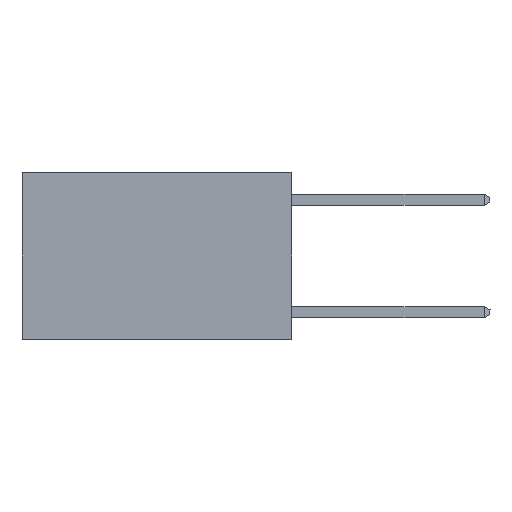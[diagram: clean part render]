
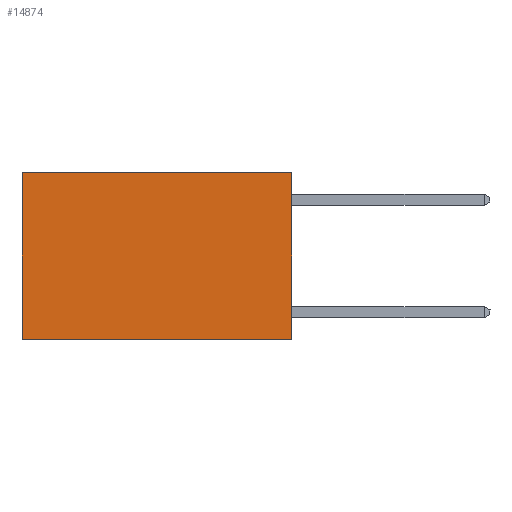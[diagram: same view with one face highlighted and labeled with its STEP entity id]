
A CAD part, left-side view. The second image highlights one B-rep face of the part: STEP entity #14874.
In plain terms, the highlighted planar face has unit normal (-1, 0, 0).
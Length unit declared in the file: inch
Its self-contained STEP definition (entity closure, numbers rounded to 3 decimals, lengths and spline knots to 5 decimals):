
#250 = CARTESIAN_POINT ( 'NONE',  ( 0.2625, 0., -0.37 ) ) ;
#368 = AXIS2_PLACEMENT_3D ( 'NONE', #15820, #8457, #18612 ) ;
#1188 = CARTESIAN_POINT ( 'NONE',  ( 0.2625, 0., 0. ) ) ;
#1323 = VERTEX_POINT ( 'NONE', #18005 ) ;
#1894 = VERTEX_POINT ( 'NONE', #3843 ) ;
#2519 = EDGE_CURVE ( 'NONE', #1323, #7548, #11680, .T. ) ;
#2812 = DIRECTION ( 'NONE',  ( 0., 0., -1. ) ) ;
#2916 = FACE_OUTER_BOUND ( 'NONE', #14482, .T. ) ;
#3797 = LINE ( 'NONE', #1188, #12005 ) ;
#3843 = CARTESIAN_POINT ( 'NONE',  ( 0.2625, 0.6, -0.37 ) ) ;
#4277 = VECTOR ( 'NONE', #8783, 39.37008 ) ;
#4704 = DIRECTION ( 'NONE',  ( 0., 1., 0. ) ) ;
#6889 = PLANE ( 'NONE',  #368 ) ;
#7424 = EDGE_CURVE ( 'NONE', #7548, #1894, #12476, .T. ) ;
#7445 = EDGE_CURVE ( 'NONE', #1323, #9102, #3797, .T. ) ;
#7548 = VERTEX_POINT ( 'NONE', #17893 ) ;
#8457 = DIRECTION ( 'NONE',  ( 1., 0., 0. ) ) ;
#8783 = DIRECTION ( 'NONE',  ( 0., 0., -1. ) ) ;
#9102 = VERTEX_POINT ( 'NONE', #250 ) ;
#10456 = LINE ( 'NONE', #12379, #11907 ) ;
#11596 = DIRECTION ( 'NONE',  ( 0., 1., 0. ) ) ;
#11680 = LINE ( 'NONE', #16669, #18368 ) ;
#11907 = VECTOR ( 'NONE', #4704, 39.37008 ) ;
#11990 = CARTESIAN_POINT ( 'NONE',  ( 0.2625, 0.6, 0. ) ) ;
#12005 = VECTOR ( 'NONE', #2812, 39.37008 ) ;
#12379 = CARTESIAN_POINT ( 'NONE',  ( 0.2625, 0., -0.37 ) ) ;
#12476 = LINE ( 'NONE', #11990, #4277 ) ;
#13282 = EDGE_CURVE ( 'NONE', #9102, #1894, #10456, .T. ) ;
#14482 = EDGE_LOOP ( 'NONE', ( #14513, #14607, #14644, #14797 ) ) ;
#14513 = ORIENTED_EDGE ( 'NONE', *, *, #7424, .T. ) ;
#14607 = ORIENTED_EDGE ( 'NONE', *, *, #13282, .F. ) ;
#14644 = ORIENTED_EDGE ( 'NONE', *, *, #7445, .F. ) ;
#14797 = ORIENTED_EDGE ( 'NONE', *, *, #2519, .T. ) ;
#14874 = ADVANCED_FACE ( 'NONE', ( #2916 ), #6889, .F. ) ;
#15820 = CARTESIAN_POINT ( 'NONE',  ( 0.2625, 0., 0. ) ) ;
#16669 = CARTESIAN_POINT ( 'NONE',  ( 0.2625, 0., 0. ) ) ;
#17893 = CARTESIAN_POINT ( 'NONE',  ( 0.2625, 0.6, 0. ) ) ;
#18005 = CARTESIAN_POINT ( 'NONE',  ( 0.2625, 0., 0. ) ) ;
#18368 = VECTOR ( 'NONE', #11596, 39.37008 ) ;
#18612 = DIRECTION ( 'NONE',  ( 0., 0., -1. ) ) ;
